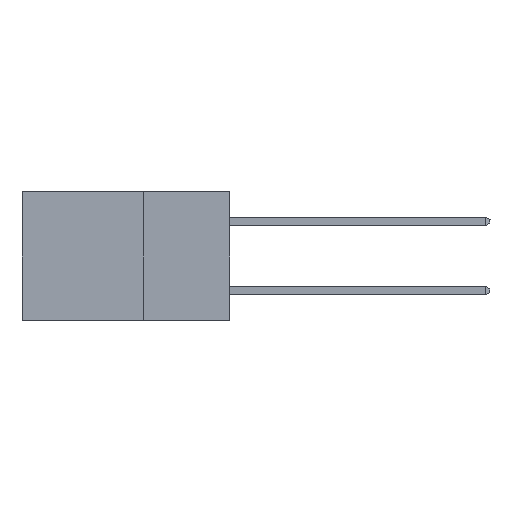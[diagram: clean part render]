
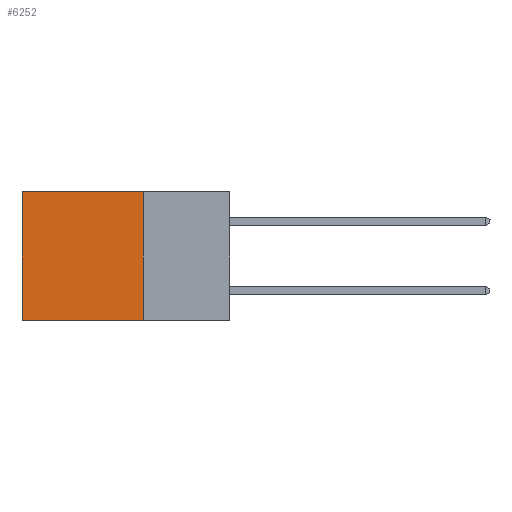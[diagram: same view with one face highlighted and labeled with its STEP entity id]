
A CAD part, left-side view. The second image highlights one B-rep face of the part: STEP entity #6252.
In plain terms, the highlighted planar face has unit normal (-1, 0, 0).
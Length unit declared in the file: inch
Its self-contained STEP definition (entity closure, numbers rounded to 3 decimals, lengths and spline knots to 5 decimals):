
#229 = DIRECTION ( 'NONE',  ( 0., 1., 0. ) ) ;
#786 = DIRECTION ( 'NONE',  ( 1., 0., 0. ) ) ;
#902 = DIRECTION ( 'NONE',  ( 0., 0., -1. ) ) ;
#1020 = CARTESIAN_POINT ( 'NONE',  ( 0.2615, 0.25, 0. ) ) ;
#1075 = CARTESIAN_POINT ( 'NONE',  ( 0.2615, 0.25, -0.37 ) ) ;
#1150 = EDGE_CURVE ( 'NONE', #5006, #6993, #2956, .T. ) ;
#1343 = VECTOR ( 'NONE', #5511, 39.37008 ) ;
#1593 = PLANE ( 'NONE',  #4236 ) ;
#2096 = LINE ( 'NONE', #8645, #1343 ) ;
#2263 = ORIENTED_EDGE ( 'NONE', *, *, #9525, .T. ) ;
#2861 = VERTEX_POINT ( 'NONE', #9447 ) ;
#2906 = ORIENTED_EDGE ( 'NONE', *, *, #1150, .F. ) ;
#2956 = LINE ( 'NONE', #6207, #3044 ) ;
#3044 = VECTOR ( 'NONE', #7877, 39.37008 ) ;
#3259 = DIRECTION ( 'NONE',  ( 0., 0., -1. ) ) ;
#4236 = AXIS2_PLACEMENT_3D ( 'NONE', #1075, #786, #3259 ) ;
#4798 = VERTEX_POINT ( 'NONE', #8880 ) ;
#5006 = VERTEX_POINT ( 'NONE', #7031 ) ;
#5078 = LINE ( 'NONE', #5719, #6454 ) ;
#5432 = ORIENTED_EDGE ( 'NONE', *, *, #8684, .T. ) ;
#5511 = DIRECTION ( 'NONE',  ( 0., 0., -1. ) ) ;
#5719 = CARTESIAN_POINT ( 'NONE',  ( 0.2615, 0.25, -0.37 ) ) ;
#6207 = CARTESIAN_POINT ( 'NONE',  ( 0.2615, 0.25, -0.37 ) ) ;
#6252 = ADVANCED_FACE ( 'NONE', ( #7218 ), #1593, .F. ) ;
#6454 = VECTOR ( 'NONE', #902, 39.37008 ) ;
#6915 = LINE ( 'NONE', #1020, #9763 ) ;
#6993 = VERTEX_POINT ( 'NONE', #7296 ) ;
#7031 = CARTESIAN_POINT ( 'NONE',  ( 0.2615, 0.25, -0.37 ) ) ;
#7046 = ORIENTED_EDGE ( 'NONE', *, *, #7567, .F. ) ;
#7218 = FACE_OUTER_BOUND ( 'NONE', #7334, .T. ) ;
#7296 = CARTESIAN_POINT ( 'NONE',  ( 0.2615, 0.6, -0.37 ) ) ;
#7334 = EDGE_LOOP ( 'NONE', ( #5432, #2906, #7046, #2263 ) ) ;
#7567 = EDGE_CURVE ( 'NONE', #4798, #5006, #5078, .T. ) ;
#7877 = DIRECTION ( 'NONE',  ( 0., 1., 0. ) ) ;
#8645 = CARTESIAN_POINT ( 'NONE',  ( 0.2615, 0.6, -0.37 ) ) ;
#8684 = EDGE_CURVE ( 'NONE', #2861, #6993, #2096, .T. ) ;
#8880 = CARTESIAN_POINT ( 'NONE',  ( 0.2615, 0.25, 0. ) ) ;
#9447 = CARTESIAN_POINT ( 'NONE',  ( 0.2615, 0.6, 0. ) ) ;
#9525 = EDGE_CURVE ( 'NONE', #4798, #2861, #6915, .T. ) ;
#9763 = VECTOR ( 'NONE', #229, 39.37008 ) ;
